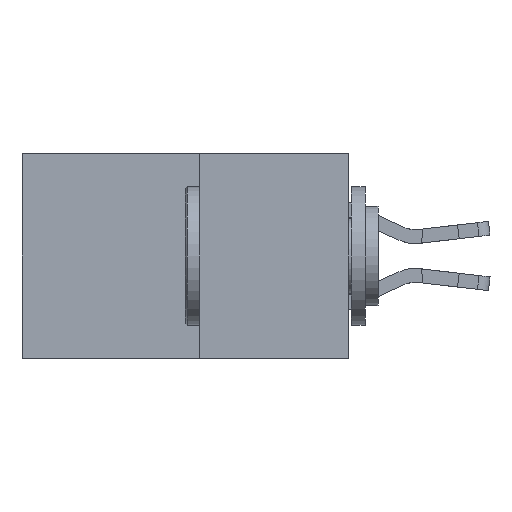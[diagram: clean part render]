
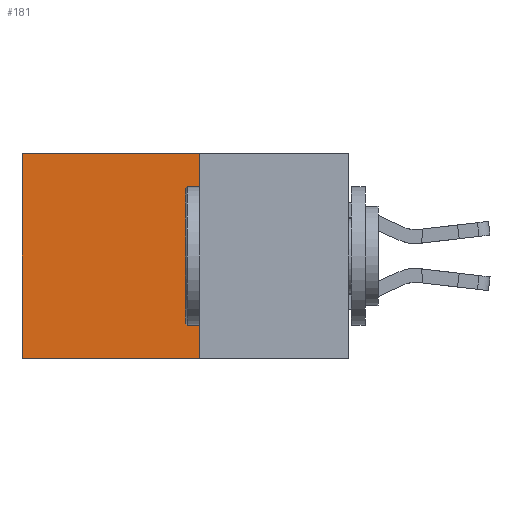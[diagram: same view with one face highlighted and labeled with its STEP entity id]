
A CAD part, left-side view. The second image highlights one B-rep face of the part: STEP entity #181.
In plain terms, the highlighted planar face has unit normal (-1, 0, 0).
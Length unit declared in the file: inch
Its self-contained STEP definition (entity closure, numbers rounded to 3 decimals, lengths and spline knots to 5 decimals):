
#181 = ADVANCED_FACE ( 'NONE', ( #526 ), #11327, .F. ) ;
#187 = DIRECTION ( 'NONE',  ( 0., 0., -1. ) ) ;
#337 = CARTESIAN_POINT ( 'NONE',  ( 0.277, 0.59, -0.37 ) ) ;
#526 = FACE_OUTER_BOUND ( 'NONE', #15628, .T. ) ;
#831 = VECTOR ( 'NONE', #3537, 39.37008 ) ;
#981 = EDGE_CURVE ( 'NONE', #2312, #16876, #8526, .T. ) ;
#1469 = ORIENTED_EDGE ( 'NONE', *, *, #981, .F. ) ;
#1609 = CARTESIAN_POINT ( 'NONE',  ( 0.277, 0.27, -0.37 ) ) ;
#1941 = VECTOR ( 'NONE', #5279, 39.37008 ) ;
#2312 = VERTEX_POINT ( 'NONE', #13667 ) ;
#3404 = ORIENTED_EDGE ( 'NONE', *, *, #5588, .T. ) ;
#3537 = DIRECTION ( 'NONE',  ( 0., 1., 0. ) ) ;
#4159 = LINE ( 'NONE', #4175, #831 ) ;
#4175 = CARTESIAN_POINT ( 'NONE',  ( 0.277, 0.27, -0.37 ) ) ;
#4324 = LINE ( 'NONE', #337, #15525 ) ;
#5048 = VERTEX_POINT ( 'NONE', #14221 ) ;
#5279 = DIRECTION ( 'NONE',  ( 0., 1., 0. ) ) ;
#5341 = CARTESIAN_POINT ( 'NONE',  ( 0.277, 0.27, 0. ) ) ;
#5588 = EDGE_CURVE ( 'NONE', #2312, #11172, #16905, .T. ) ;
#5938 = AXIS2_PLACEMENT_3D ( 'NONE', #11170, #11047, #11369 ) ;
#6377 = EDGE_CURVE ( 'NONE', #16876, #5048, #4159, .T. ) ;
#7608 = ORIENTED_EDGE ( 'NONE', *, *, #6377, .F. ) ;
#7959 = EDGE_CURVE ( 'NONE', #11172, #5048, #4324, .T. ) ;
#8526 = LINE ( 'NONE', #16404, #11799 ) ;
#9297 = ORIENTED_EDGE ( 'NONE', *, *, #7959, .T. ) ;
#11047 = DIRECTION ( 'NONE',  ( 1., 0., 0. ) ) ;
#11170 = CARTESIAN_POINT ( 'NONE',  ( 0.277, 0.27, -0.37 ) ) ;
#11172 = VERTEX_POINT ( 'NONE', #13684 ) ;
#11327 = PLANE ( 'NONE',  #5938 ) ;
#11369 = DIRECTION ( 'NONE',  ( 0., 0., -1. ) ) ;
#11799 = VECTOR ( 'NONE', #13581, 39.37008 ) ;
#13581 = DIRECTION ( 'NONE',  ( 0., 0., -1. ) ) ;
#13667 = CARTESIAN_POINT ( 'NONE',  ( 0.277, 0.27, 0. ) ) ;
#13684 = CARTESIAN_POINT ( 'NONE',  ( 0.277, 0.59, 0. ) ) ;
#14221 = CARTESIAN_POINT ( 'NONE',  ( 0.277, 0.59, -0.37 ) ) ;
#15525 = VECTOR ( 'NONE', #187, 39.37008 ) ;
#15628 = EDGE_LOOP ( 'NONE', ( #9297, #7608, #1469, #3404 ) ) ;
#16404 = CARTESIAN_POINT ( 'NONE',  ( 0.277, 0.27, -0.37 ) ) ;
#16876 = VERTEX_POINT ( 'NONE', #1609 ) ;
#16905 = LINE ( 'NONE', #5341, #1941 ) ;
